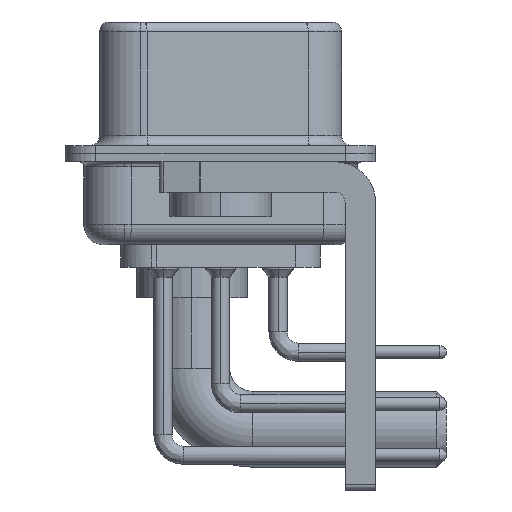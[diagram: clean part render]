
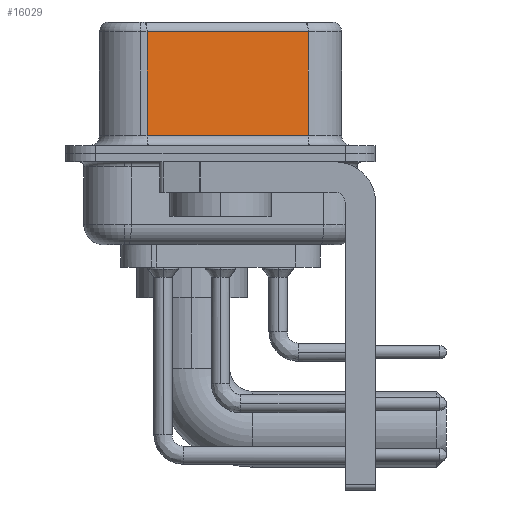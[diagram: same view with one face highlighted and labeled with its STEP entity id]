
A CAD part, left-side view. The second image highlights one B-rep face of the part: STEP entity #16029.
In plain terms, the highlighted planar face has unit normal (-0.985, -0.174, 0).
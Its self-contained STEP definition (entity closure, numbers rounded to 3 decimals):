
#1283 = LINE ( 'NONE', #14011, #37744 ) ;
#2587 = DIRECTION ( 'NONE',  ( 0.174, -0.985, 0. ) ) ;
#4332 = PLANE ( 'NONE',  #37982 ) ;
#5109 = EDGE_LOOP ( 'NONE', ( #14954, #13201, #16735, #17742 ) ) ;
#6030 = DIRECTION ( 'NONE',  ( 0., 0., -1. ) ) ;
#10502 = DIRECTION ( 'NONE',  ( -0.174, 0.985, 0. ) ) ;
#10861 = EDGE_CURVE ( 'NONE', #17114, #18219, #1283, .T. ) ;
#13133 = VERTEX_POINT ( 'NONE', #19106 ) ;
#13201 = ORIENTED_EDGE ( 'NONE', *, *, #33235, .T. ) ;
#14011 = CARTESIAN_POINT ( 'NONE',  ( 5.132, -4.322, 0.9 ) ) ;
#14954 = ORIENTED_EDGE ( 'NONE', *, *, #27362, .F. ) ;
#16029 = ADVANCED_FACE ( 'NONE', ( #36528 ), #4332, .F. ) ;
#16735 = ORIENTED_EDGE ( 'NONE', *, *, #21669, .T. ) ;
#17114 = VERTEX_POINT ( 'NONE', #22458 ) ;
#17742 = ORIENTED_EDGE ( 'NONE', *, *, #10861, .T. ) ;
#18219 = VERTEX_POINT ( 'NONE', #33521 ) ;
#18302 = CARTESIAN_POINT ( 'NONE',  ( 5.132, -4.322, 6.52 ) ) ;
#18874 = DIRECTION ( 'NONE',  ( -0.174, 0.985, 0. ) ) ;
#19106 = CARTESIAN_POINT ( 'NONE',  ( 5.132, -4.322, 6.02 ) ) ;
#19415 = LINE ( 'NONE', #33959, #32080 ) ;
#21669 = EDGE_CURVE ( 'NONE', #31460, #17114, #24580, .T. ) ;
#21782 = CARTESIAN_POINT ( 'NONE',  ( 5.132, -4.322, 6.52 ) ) ;
#22090 = VECTOR ( 'NONE', #30141, 1000. ) ;
#22458 = CARTESIAN_POINT ( 'NONE',  ( 3.73, 3.628, 0.9 ) ) ;
#24580 = LINE ( 'NONE', #24772, #34189 ) ;
#24772 = CARTESIAN_POINT ( 'NONE',  ( 3.73, 3.628, 6.52 ) ) ;
#27362 = EDGE_CURVE ( 'NONE', #13133, #18219, #33033, .T. ) ;
#30141 = DIRECTION ( 'NONE',  ( 0., 0., -1. ) ) ;
#31460 = VERTEX_POINT ( 'NONE', #35778 ) ;
#32080 = VECTOR ( 'NONE', #10502, 1000. ) ;
#33033 = LINE ( 'NONE', #18302, #22090 ) ;
#33235 = EDGE_CURVE ( 'NONE', #13133, #31460, #19415, .T. ) ;
#33521 = CARTESIAN_POINT ( 'NONE',  ( 5.132, -4.322, 0.9 ) ) ;
#33606 = DIRECTION ( 'NONE',  ( 0.985, 0.174, 0. ) ) ;
#33959 = CARTESIAN_POINT ( 'NONE',  ( 5.132, -4.322, 6.02 ) ) ;
#34189 = VECTOR ( 'NONE', #6030, 1000. ) ;
#35778 = CARTESIAN_POINT ( 'NONE',  ( 3.73, 3.628, 6.02 ) ) ;
#36528 = FACE_OUTER_BOUND ( 'NONE', #5109, .T. ) ;
#37744 = VECTOR ( 'NONE', #2587, 1000. ) ;
#37982 = AXIS2_PLACEMENT_3D ( 'NONE', #21782, #33606, #18874 ) ;
